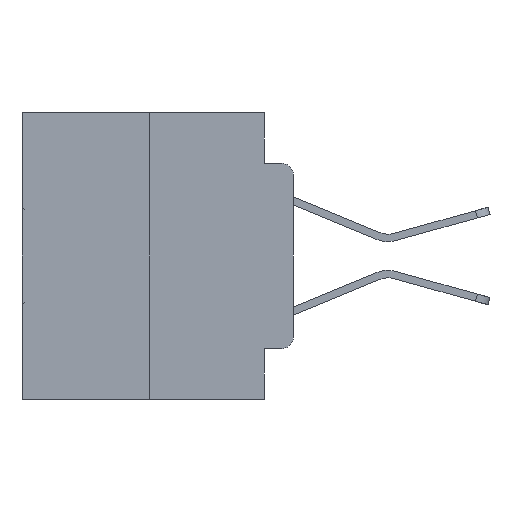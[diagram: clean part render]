
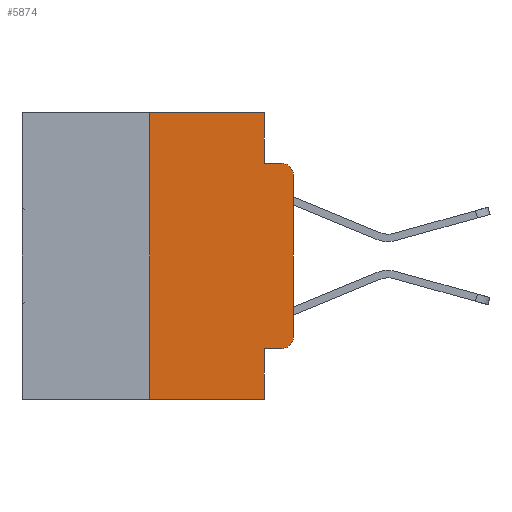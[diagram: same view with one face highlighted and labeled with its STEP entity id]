
A CAD part, left-side view. The second image highlights one B-rep face of the part: STEP entity #5874.
In plain terms, the highlighted planar face has unit normal (-1, 0, 0).
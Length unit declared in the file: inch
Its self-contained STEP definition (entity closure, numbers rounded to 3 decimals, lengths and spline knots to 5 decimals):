
#673 = VERTEX_POINT ( 'NONE', #21507 ) ;
#1133 = EDGE_CURVE ( 'NONE', #22236, #15242, #2385, .T. ) ;
#1224 = DIRECTION ( 'NONE',  ( 0., -1., 0. ) ) ;
#1581 = CIRCLE ( 'NONE', #6667, 0.02 ) ;
#1675 = CARTESIAN_POINT ( 'NONE',  ( 0., 0.051, -0.0885 ) ) ;
#2385 = LINE ( 'NONE', #24573, #5239 ) ;
#3171 = DIRECTION ( 'NONE',  ( 0., -1., 0. ) ) ;
#3219 = CARTESIAN_POINT ( 'NONE',  ( 0., 0.02, -0.0885 ) ) ;
#3729 = VECTOR ( 'NONE', #30359, 39.37008 ) ;
#3802 = CARTESIAN_POINT ( 'NONE',  ( 0., 0.473, 0. ) ) ;
#4169 = VECTOR ( 'NONE', #7236, 39.37008 ) ;
#4429 = CIRCLE ( 'NONE', #19105, 0.02 ) ;
#4591 = CARTESIAN_POINT ( 'NONE',  ( 0., 0.051, 0. ) ) ;
#4927 = EDGE_CURVE ( 'NONE', #21287, #25445, #8680, .T. ) ;
#5166 = AXIS2_PLACEMENT_3D ( 'NONE', #31060, #26179, #16344 ) ;
#5239 = VECTOR ( 'NONE', #7481, 39.37008 ) ;
#5398 = CARTESIAN_POINT ( 'NONE',  ( 0., 0.051, 0. ) ) ;
#5706 = ORIENTED_EDGE ( 'NONE', *, *, #7448, .F. ) ;
#5715 = LINE ( 'NONE', #22963, #28551 ) ;
#5874 = ADVANCED_FACE ( 'NONE', ( #6701 ), #16501, .F. ) ;
#5949 = ORIENTED_EDGE ( 'NONE', *, *, #10662, .F. ) ;
#6556 = CARTESIAN_POINT ( 'NONE',  ( 0., 0., -0.1085 ) ) ;
#6667 = AXIS2_PLACEMENT_3D ( 'NONE', #11740, #11425, #16331 ) ;
#6701 = FACE_OUTER_BOUND ( 'NONE', #29835, .T. ) ;
#7236 = DIRECTION ( 'NONE',  ( 0., 0., -1. ) ) ;
#7448 = EDGE_CURVE ( 'NONE', #25863, #25233, #18077, .T. ) ;
#7481 = DIRECTION ( 'NONE',  ( 0., 0., 1. ) ) ;
#8113 = CARTESIAN_POINT ( 'NONE',  ( 0., 0., -0.3915 ) ) ;
#8368 = VECTOR ( 'NONE', #30369, 39.37008 ) ;
#8680 = LINE ( 'NONE', #15483, #3729 ) ;
#8814 = DIRECTION ( 'NONE',  ( 0., 0., -1. ) ) ;
#9355 = DIRECTION ( 'NONE',  ( 0., 0., -1. ) ) ;
#9379 = ORIENTED_EDGE ( 'NONE', *, *, #10459, .T. ) ;
#10429 = VERTEX_POINT ( 'NONE', #5398 ) ;
#10459 = EDGE_CURVE ( 'NONE', #673, #26629, #5715, .T. ) ;
#10551 = EDGE_CURVE ( 'NONE', #15242, #10429, #10931, .T. ) ;
#10662 = EDGE_CURVE ( 'NONE', #673, #13266, #21075, .T. ) ;
#10931 = LINE ( 'NONE', #3802, #25506 ) ;
#11425 = DIRECTION ( 'NONE',  ( -1., 0., 0. ) ) ;
#11665 = ORIENTED_EDGE ( 'NONE', *, *, #10551, .F. ) ;
#11740 = CARTESIAN_POINT ( 'NONE',  ( 0., 0.02, -0.1085 ) ) ;
#13141 = EDGE_CURVE ( 'NONE', #26629, #21287, #4429, .T. ) ;
#13266 = VERTEX_POINT ( 'NONE', #21331 ) ;
#13583 = VECTOR ( 'NONE', #29619, 39.37008 ) ;
#14166 = CARTESIAN_POINT ( 'NONE',  ( 0., 0.02, -0.4115 ) ) ;
#14212 = DIRECTION ( 'NONE',  ( -1., 0., 0. ) ) ;
#14674 = CARTESIAN_POINT ( 'NONE',  ( 0., 0.051, 0. ) ) ;
#15242 = VERTEX_POINT ( 'NONE', #25213 ) ;
#15483 = CARTESIAN_POINT ( 'NONE',  ( 0., 0., 0. ) ) ;
#16331 = DIRECTION ( 'NONE',  ( 0., 0., -1. ) ) ;
#16344 = DIRECTION ( 'NONE',  ( 0., 0., -1. ) ) ;
#16501 = PLANE ( 'NONE',  #5166 ) ;
#18077 = LINE ( 'NONE', #20616, #13583 ) ;
#19105 = AXIS2_PLACEMENT_3D ( 'NONE', #28605, #14212, #8814 ) ;
#19306 = EDGE_CURVE ( 'NONE', #25445, #25233, #1581, .T. ) ;
#20344 = EDGE_CURVE ( 'NONE', #10429, #25863, #26704, .T. ) ;
#20616 = CARTESIAN_POINT ( 'NONE',  ( 0., 0.051, -0.0885 ) ) ;
#21075 = LINE ( 'NONE', #4591, #27568 ) ;
#21287 = VERTEX_POINT ( 'NONE', #8113 ) ;
#21331 = CARTESIAN_POINT ( 'NONE',  ( 0., 0.051, -0.5 ) ) ;
#21507 = CARTESIAN_POINT ( 'NONE',  ( 0., 0.051, -0.4115 ) ) ;
#21930 = EDGE_CURVE ( 'NONE', #22236, #13266, #23089, .T. ) ;
#22175 = ORIENTED_EDGE ( 'NONE', *, *, #19306, .T. ) ;
#22236 = VERTEX_POINT ( 'NONE', #24349 ) ;
#22664 = ORIENTED_EDGE ( 'NONE', *, *, #21930, .T. ) ;
#22963 = CARTESIAN_POINT ( 'NONE',  ( 0., 0.051, -0.4115 ) ) ;
#23089 = LINE ( 'NONE', #27391, #8368 ) ;
#24349 = CARTESIAN_POINT ( 'NONE',  ( 0., 0.25, -0.5 ) ) ;
#24573 = CARTESIAN_POINT ( 'NONE',  ( 0., 0.25, 0. ) ) ;
#25213 = CARTESIAN_POINT ( 'NONE',  ( 0., 0.25, 0. ) ) ;
#25233 = VERTEX_POINT ( 'NONE', #3219 ) ;
#25445 = VERTEX_POINT ( 'NONE', #6556 ) ;
#25506 = VECTOR ( 'NONE', #3171, 39.37008 ) ;
#25863 = VERTEX_POINT ( 'NONE', #1675 ) ;
#26079 = ORIENTED_EDGE ( 'NONE', *, *, #13141, .T. ) ;
#26179 = DIRECTION ( 'NONE',  ( 1., 0., 0. ) ) ;
#26604 = ORIENTED_EDGE ( 'NONE', *, *, #1133, .F. ) ;
#26629 = VERTEX_POINT ( 'NONE', #14166 ) ;
#26657 = ORIENTED_EDGE ( 'NONE', *, *, #20344, .F. ) ;
#26704 = LINE ( 'NONE', #14674, #4169 ) ;
#26849 = ORIENTED_EDGE ( 'NONE', *, *, #4927, .T. ) ;
#27391 = CARTESIAN_POINT ( 'NONE',  ( 0., 0.473, -0.5 ) ) ;
#27568 = VECTOR ( 'NONE', #9355, 39.37008 ) ;
#28551 = VECTOR ( 'NONE', #1224, 39.37008 ) ;
#28605 = CARTESIAN_POINT ( 'NONE',  ( 0., 0.02, -0.3915 ) ) ;
#29619 = DIRECTION ( 'NONE',  ( 0., -1., 0. ) ) ;
#29835 = EDGE_LOOP ( 'NONE', ( #26849, #22175, #5706, #26657, #11665, #26604, #22664, #5949, #9379, #26079 ) ) ;
#30359 = DIRECTION ( 'NONE',  ( 0., 0., 1. ) ) ;
#30369 = DIRECTION ( 'NONE',  ( 0., -1., 0. ) ) ;
#31060 = CARTESIAN_POINT ( 'NONE',  ( 0., 0.473, 0. ) ) ;
